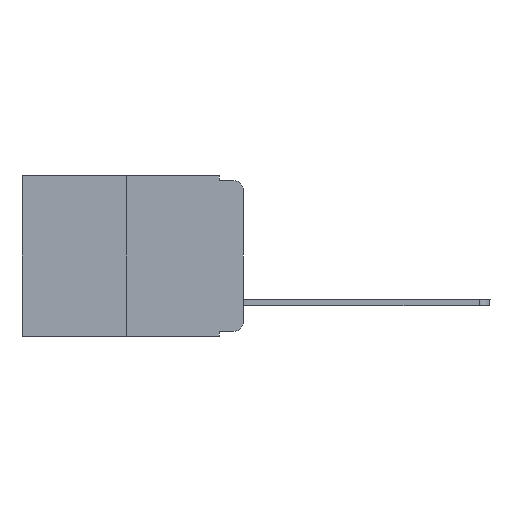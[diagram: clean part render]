
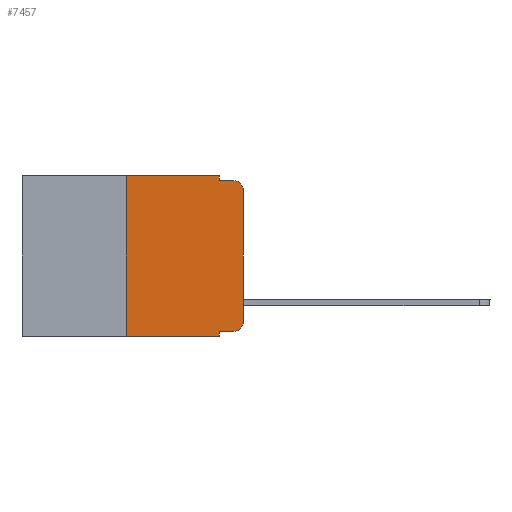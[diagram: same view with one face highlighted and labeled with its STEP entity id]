
A CAD part, left-side view. The second image highlights one B-rep face of the part: STEP entity #7457.
In plain terms, the highlighted planar face has unit normal (-1, 0, 0).
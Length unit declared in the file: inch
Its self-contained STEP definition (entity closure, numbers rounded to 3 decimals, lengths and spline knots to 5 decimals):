
#260 = DIRECTION ( 'NONE',  ( 0., -1., 0. ) ) ;
#788 = CARTESIAN_POINT ( 'NONE',  ( 0., 0.25, -0.343 ) ) ;
#824 = DIRECTION ( 'NONE',  ( -1., 0., 0. ) ) ;
#832 = CARTESIAN_POINT ( 'NONE',  ( 0., 0., -0.313 ) ) ;
#1091 = AXIS2_PLACEMENT_3D ( 'NONE', #18003, #824, #12317 ) ;
#1228 = AXIS2_PLACEMENT_3D ( 'NONE', #1827, #9535, #15343 ) ;
#1827 = CARTESIAN_POINT ( 'NONE',  ( 0., 0.473, 0. ) ) ;
#2250 = EDGE_LOOP ( 'NONE', ( #2324, #11895, #6669, #10514, #8722, #3757, #16328, #5148, #13982, #6653 ) ) ;
#2285 = EDGE_CURVE ( 'NONE', #18475, #17897, #8747, .T. ) ;
#2309 = CARTESIAN_POINT ( 'NONE',  ( 0., 0.051, 0. ) ) ;
#2324 = ORIENTED_EDGE ( 'NONE', *, *, #8586, .T. ) ;
#3430 = CARTESIAN_POINT ( 'NONE',  ( 0., 0.02, -0.03 ) ) ;
#3682 = EDGE_CURVE ( 'NONE', #23479, #14750, #14120, .T. ) ;
#3757 = ORIENTED_EDGE ( 'NONE', *, *, #3682, .F. ) ;
#4700 = DIRECTION ( 'NONE',  ( 0., 0., -1. ) ) ;
#5148 = ORIENTED_EDGE ( 'NONE', *, *, #14774, .F. ) ;
#5230 = FACE_OUTER_BOUND ( 'NONE', #2250, .T. ) ;
#5251 = DIRECTION ( 'NONE',  ( 0., -1., 0. ) ) ;
#5945 = CARTESIAN_POINT ( 'NONE',  ( 0., 0.051, -0.343 ) ) ;
#6103 = CARTESIAN_POINT ( 'NONE',  ( 0., 0.02, -0.333 ) ) ;
#6196 = VERTEX_POINT ( 'NONE', #5945 ) ;
#6649 = CARTESIAN_POINT ( 'NONE',  ( 0., 0.25, 0. ) ) ;
#6653 = ORIENTED_EDGE ( 'NONE', *, *, #2285, .T. ) ;
#6669 = ORIENTED_EDGE ( 'NONE', *, *, #9455, .F. ) ;
#7457 = ADVANCED_FACE ( 'NONE', ( #5230 ), #19135, .F. ) ;
#7684 = LINE ( 'NONE', #22843, #8167 ) ;
#7907 = EDGE_CURVE ( 'NONE', #20043, #20504, #22608, .T. ) ;
#8013 = CARTESIAN_POINT ( 'NONE',  ( 0., 0.051, -0.333 ) ) ;
#8167 = VECTOR ( 'NONE', #20959, 39.37008 ) ;
#8586 = EDGE_CURVE ( 'NONE', #17897, #20043, #14471, .T. ) ;
#8722 = ORIENTED_EDGE ( 'NONE', *, *, #17670, .F. ) ;
#8747 = CIRCLE ( 'NONE', #1091, 0.02 ) ;
#9134 = DIRECTION ( 'NONE',  ( 0., 0., -1. ) ) ;
#9455 = EDGE_CURVE ( 'NONE', #24952, #20504, #7684, .T. ) ;
#9535 = DIRECTION ( 'NONE',  ( 1., 0., 0. ) ) ;
#10129 = CARTESIAN_POINT ( 'NONE',  ( 0., 0., -0.03 ) ) ;
#10233 = CARTESIAN_POINT ( 'NONE',  ( 0., 0.051, -0.333 ) ) ;
#10236 = DIRECTION ( 'NONE',  ( 0., -1., 0. ) ) ;
#10292 = VECTOR ( 'NONE', #260, 39.37008 ) ;
#10514 = ORIENTED_EDGE ( 'NONE', *, *, #12357, .F. ) ;
#10681 = CARTESIAN_POINT ( 'NONE',  ( 0., 0., 0. ) ) ;
#10806 = VECTOR ( 'NONE', #22310, 39.37008 ) ;
#11463 = VECTOR ( 'NONE', #4700, 39.37008 ) ;
#11621 = EDGE_CURVE ( 'NONE', #23479, #6196, #12254, .T. ) ;
#11734 = AXIS2_PLACEMENT_3D ( 'NONE', #3430, #24413, #9134 ) ;
#11895 = ORIENTED_EDGE ( 'NONE', *, *, #7907, .T. ) ;
#12238 = CARTESIAN_POINT ( 'NONE',  ( 0., 0.02, -0.01 ) ) ;
#12254 = LINE ( 'NONE', #21482, #14231 ) ;
#12317 = DIRECTION ( 'NONE',  ( 0., 0., -1. ) ) ;
#12357 = EDGE_CURVE ( 'NONE', #17840, #24952, #14184, .T. ) ;
#12596 = CARTESIAN_POINT ( 'NONE',  ( 0., 0.473, 0. ) ) ;
#13148 = VECTOR ( 'NONE', #5251, 39.37008 ) ;
#13982 = ORIENTED_EDGE ( 'NONE', *, *, #14975, .T. ) ;
#14120 = LINE ( 'NONE', #6649, #10806 ) ;
#14184 = LINE ( 'NONE', #2309, #11463 ) ;
#14231 = VECTOR ( 'NONE', #10236, 39.37008 ) ;
#14471 = LINE ( 'NONE', #10681, #21825 ) ;
#14750 = VERTEX_POINT ( 'NONE', #18454 ) ;
#14774 = EDGE_CURVE ( 'NONE', #21821, #6196, #16568, .T. ) ;
#14975 = EDGE_CURVE ( 'NONE', #21821, #18475, #23373, .T. ) ;
#15343 = DIRECTION ( 'NONE',  ( 0., 0., -1. ) ) ;
#16328 = ORIENTED_EDGE ( 'NONE', *, *, #11621, .T. ) ;
#16445 = CARTESIAN_POINT ( 'NONE',  ( 0., 0.051, -0.01 ) ) ;
#16568 = LINE ( 'NONE', #24268, #24906 ) ;
#16690 = DIRECTION ( 'NONE',  ( 0., 0., -1. ) ) ;
#17670 = EDGE_CURVE ( 'NONE', #14750, #17840, #24463, .T. ) ;
#17840 = VERTEX_POINT ( 'NONE', #19281 ) ;
#17897 = VERTEX_POINT ( 'NONE', #832 ) ;
#18003 = CARTESIAN_POINT ( 'NONE',  ( 0., 0.02, -0.313 ) ) ;
#18454 = CARTESIAN_POINT ( 'NONE',  ( 0., 0.25, 0. ) ) ;
#18475 = VERTEX_POINT ( 'NONE', #6103 ) ;
#19135 = PLANE ( 'NONE',  #1228 ) ;
#19281 = CARTESIAN_POINT ( 'NONE',  ( 0., 0.051, 0. ) ) ;
#20043 = VERTEX_POINT ( 'NONE', #10129 ) ;
#20504 = VERTEX_POINT ( 'NONE', #12238 ) ;
#20959 = DIRECTION ( 'NONE',  ( 0., -1., 0. ) ) ;
#21482 = CARTESIAN_POINT ( 'NONE',  ( 0., 0.473, -0.343 ) ) ;
#21821 = VERTEX_POINT ( 'NONE', #8013 ) ;
#21825 = VECTOR ( 'NONE', #24195, 39.37008 ) ;
#22310 = DIRECTION ( 'NONE',  ( 0., 0., 1. ) ) ;
#22608 = CIRCLE ( 'NONE', #11734, 0.02 ) ;
#22843 = CARTESIAN_POINT ( 'NONE',  ( 0., 0.051, -0.01 ) ) ;
#23373 = LINE ( 'NONE', #10233, #10292 ) ;
#23479 = VERTEX_POINT ( 'NONE', #788 ) ;
#24195 = DIRECTION ( 'NONE',  ( 0., 0., 1. ) ) ;
#24268 = CARTESIAN_POINT ( 'NONE',  ( 0., 0.051, 0. ) ) ;
#24413 = DIRECTION ( 'NONE',  ( -1., 0., 0. ) ) ;
#24463 = LINE ( 'NONE', #12596, #13148 ) ;
#24906 = VECTOR ( 'NONE', #16690, 39.37008 ) ;
#24952 = VERTEX_POINT ( 'NONE', #16445 ) ;
